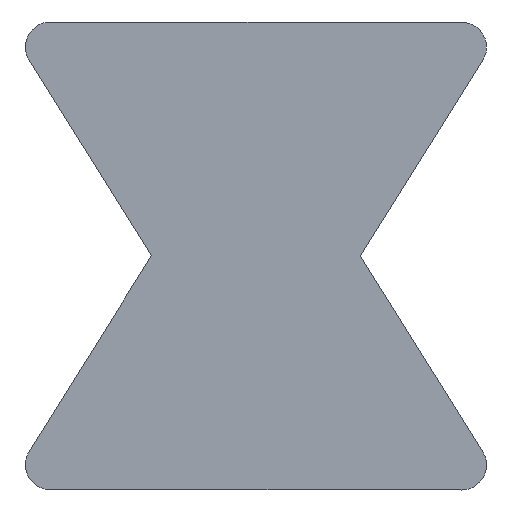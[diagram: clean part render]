
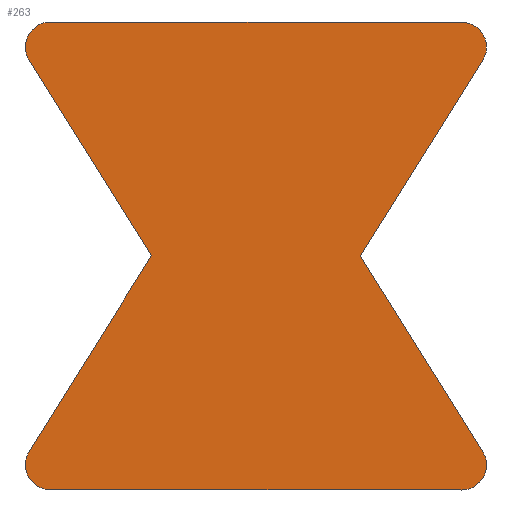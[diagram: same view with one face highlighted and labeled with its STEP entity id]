
A CAD part, front view. The second image highlights one B-rep face of the part: STEP entity #263.
In plain terms, the highlighted planar face has unit normal (0, -1, 0).
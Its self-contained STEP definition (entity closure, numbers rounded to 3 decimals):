
#16=CIRCLE('',#282,1.);
#18=CIRCLE('',#286,1.);
#20=CIRCLE('',#289,1.);
#22=CIRCLE('',#295,1.);
#24=CIRCLE('',#299,1.);
#42=FACE_OUTER_BOUND('',#56,.T.);
#56=EDGE_LOOP('',(#218,#219,#220,#221,#222,#223,#224,#225,#226,#227,#228,
#229));
#60=LINE('',#387,#86);
#64=LINE('',#399,#90);
#69=LINE('',#417,#95);
#72=LINE('',#423,#98);
#75=LINE('',#429,#101);
#79=LINE('',#441,#105);
#83=LINE('',#451,#109);
#86=VECTOR('',#309,10.);
#90=VECTOR('',#321,10.);
#95=VECTOR('',#340,10.);
#98=VECTOR('',#345,10.);
#101=VECTOR('',#350,10.);
#105=VECTOR('',#362,10.);
#109=VECTOR('',#374,10.);
#112=VERTEX_POINT('',#384);
#113=VERTEX_POINT('',#386);
#115=VERTEX_POINT('',#392);
#117=VERTEX_POINT('',#398);
#119=VERTEX_POINT('',#404);
#121=VERTEX_POINT('',#410);
#123=VERTEX_POINT('',#416);
#125=VERTEX_POINT('',#422);
#127=VERTEX_POINT('',#428);
#129=VERTEX_POINT('',#434);
#131=VERTEX_POINT('',#440);
#133=VERTEX_POINT('',#446);
#136=EDGE_CURVE('',#113,#112,#60,.T.);
#139=EDGE_CURVE('',#115,#113,#16,.T.);
#142=EDGE_CURVE('',#117,#115,#64,.T.);
#145=EDGE_CURVE('',#119,#117,#18,.T.);
#148=EDGE_CURVE('',#121,#119,#20,.T.);
#151=EDGE_CURVE('',#123,#121,#69,.T.);
#154=EDGE_CURVE('',#125,#123,#72,.T.);
#157=EDGE_CURVE('',#127,#125,#75,.T.);
#160=EDGE_CURVE('',#129,#127,#22,.T.);
#163=EDGE_CURVE('',#131,#129,#79,.T.);
#166=EDGE_CURVE('',#133,#131,#24,.T.);
#169=EDGE_CURVE('',#112,#133,#83,.T.);
#218=ORIENTED_EDGE('',*,*,#169,.T.);
#219=ORIENTED_EDGE('',*,*,#166,.T.);
#220=ORIENTED_EDGE('',*,*,#163,.T.);
#221=ORIENTED_EDGE('',*,*,#160,.T.);
#222=ORIENTED_EDGE('',*,*,#157,.T.);
#223=ORIENTED_EDGE('',*,*,#154,.T.);
#224=ORIENTED_EDGE('',*,*,#151,.T.);
#225=ORIENTED_EDGE('',*,*,#148,.T.);
#226=ORIENTED_EDGE('',*,*,#145,.T.);
#227=ORIENTED_EDGE('',*,*,#142,.T.);
#228=ORIENTED_EDGE('',*,*,#139,.T.);
#229=ORIENTED_EDGE('',*,*,#136,.T.);
#249=PLANE('',#301);
#263=ADVANCED_FACE('',(#42),#249,.T.);
#282=AXIS2_PLACEMENT_3D('',#393,#315,#316);
#286=AXIS2_PLACEMENT_3D('',#405,#327,#328);
#289=AXIS2_PLACEMENT_3D('',#411,#334,#335);
#295=AXIS2_PLACEMENT_3D('',#435,#356,#357);
#299=AXIS2_PLACEMENT_3D('',#447,#368,#369);
#301=AXIS2_PLACEMENT_3D('',#452,#375,#376);
#309=DIRECTION('',(0.53,0.,-0.848));
#315=DIRECTION('center_axis',(0.,-1.,0.));
#316=DIRECTION('ref_axis',(0.,0.,1.));
#321=DIRECTION('',(-1.,0.,0.));
#327=DIRECTION('center_axis',(0.,-1.,0.));
#328=DIRECTION('ref_axis',(0.848,0.,-0.53));
#334=DIRECTION('center_axis',(0.,-1.,0.));
#335=DIRECTION('ref_axis',(0.848,0.,-0.53));
#340=DIRECTION('',(0.53,0.,0.848));
#345=DIRECTION('',(0.,0.,1.));
#350=DIRECTION('',(-0.53,0.,0.848));
#356=DIRECTION('center_axis',(0.,-1.,0.));
#357=DIRECTION('ref_axis',(0.,0.,-1.));
#362=DIRECTION('',(1.,0.,0.));
#368=DIRECTION('center_axis',(0.,-1.,0.));
#369=DIRECTION('ref_axis',(-0.848,0.,0.53));
#374=DIRECTION('',(-0.53,0.,-0.848));
#375=DIRECTION('center_axis',(0.,-1.,0.));
#376=DIRECTION('ref_axis',(1.,0.,0.));
#384=CARTESIAN_POINT('',(54.235,121.626,-87.549));
#386=CARTESIAN_POINT('',(49.362,121.626,-79.751));
#387=CARTESIAN_POINT('',(54.235,121.626,-87.549));
#392=CARTESIAN_POINT('',(50.211,121.626,-78.222));
#393=CARTESIAN_POINT('Origin',(50.21,121.626,-79.222));
#398=CARTESIAN_POINT('',(66.603,121.626,-78.23));
#399=CARTESIAN_POINT('',(66.603,121.626,-78.23));
#404=CARTESIAN_POINT('',(67.6,121.626,-79.163));
#405=CARTESIAN_POINT('Origin',(66.602,121.626,-79.23));
#410=CARTESIAN_POINT('',(67.45,121.626,-79.751));
#411=CARTESIAN_POINT('Origin',(66.602,121.626,-79.221));
#416=CARTESIAN_POINT('',(62.577,121.626,-87.549));
#417=CARTESIAN_POINT('',(62.577,121.626,-87.549));
#422=CARTESIAN_POINT('',(62.577,121.626,-87.559));
#423=CARTESIAN_POINT('',(62.577,121.626,-87.559));
#428=CARTESIAN_POINT('',(67.449,121.626,-95.357));
#429=CARTESIAN_POINT('',(62.577,121.626,-87.559));
#434=CARTESIAN_POINT('',(66.601,121.626,-96.887));
#435=CARTESIAN_POINT('Origin',(66.601,121.626,-95.887));
#440=CARTESIAN_POINT('',(50.209,121.626,-96.879));
#441=CARTESIAN_POINT('',(66.601,121.626,-96.887));
#446=CARTESIAN_POINT('',(49.361,121.626,-95.349));
#447=CARTESIAN_POINT('Origin',(50.21,121.626,-95.879));
#451=CARTESIAN_POINT('',(54.235,121.626,-87.549));
#452=CARTESIAN_POINT('Origin',(58.406,121.626,-87.554));
